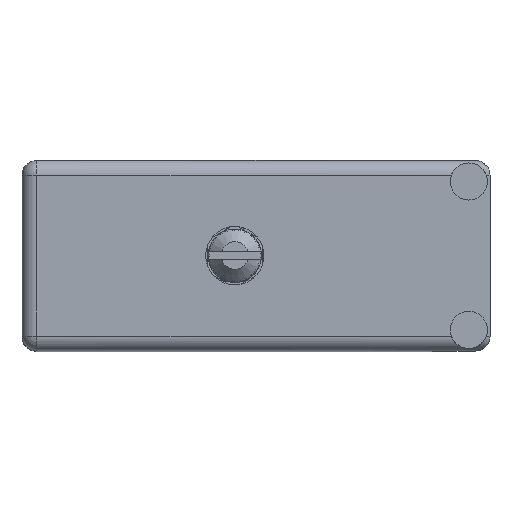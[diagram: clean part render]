
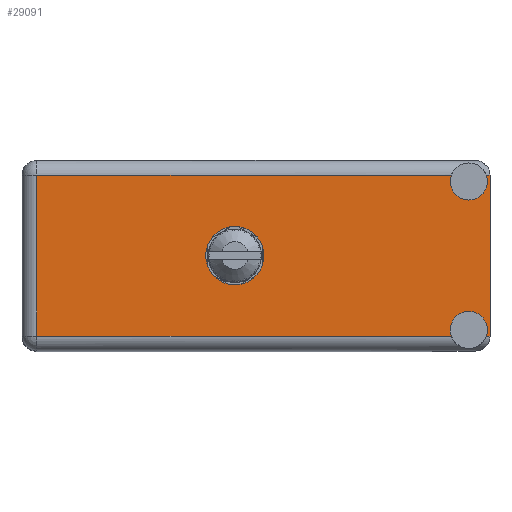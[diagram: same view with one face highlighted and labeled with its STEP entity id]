
A CAD part, top view. The second image highlights one B-rep face of the part: STEP entity #29091.
In plain terms, the highlighted face is planar.
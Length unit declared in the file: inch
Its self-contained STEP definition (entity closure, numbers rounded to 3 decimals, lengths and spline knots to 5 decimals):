
#1974 = DIRECTION ( 'NONE',  ( 0., 1., 0. ) ) ;
#2074 = AXIS2_PLACEMENT_3D ( 'NONE', #16727, #26383, #71237 ) ;
#2833 = VECTOR ( 'NONE', #26097, 39.37008 ) ;
#4726 = VERTEX_POINT ( 'NONE', #74953 ) ;
#4995 = ORIENTED_EDGE ( 'NONE', *, *, #96142, .F. ) ;
#7237 = LINE ( 'NONE', #66171, #75024 ) ;
#10432 = VERTEX_POINT ( 'NONE', #50544 ) ;
#12058 = EDGE_CURVE ( 'NONE', #27234, #93784, #113014, .T. ) ;
#13384 = EDGE_CURVE ( 'NONE', #50701, #30802, #27022, .T. ) ;
#13853 = DIRECTION ( 'NONE',  ( 0., 0., 1. ) ) ;
#14037 = DIRECTION ( 'NONE',  ( 0., 1., 0. ) ) ;
#15318 = AXIS2_PLACEMENT_3D ( 'NONE', #91038, #99223, #46219 ) ;
#15654 = ORIENTED_EDGE ( 'NONE', *, *, #12058, .T. ) ;
#16643 = ORIENTED_EDGE ( 'NONE', *, *, #84531, .F. ) ;
#16688 = DIRECTION ( 'NONE',  ( 0., 1., 0. ) ) ;
#16727 = CARTESIAN_POINT ( 'NONE',  ( 1.104, 1.466, 0.35 ) ) ;
#21860 = CIRCLE ( 'NONE', #15318, 0.1375 ) ;
#23743 = CARTESIAN_POINT ( 'NONE',  ( -1.004, 1.466, -0.4495 ) ) ;
#23768 = ORIENTED_EDGE ( 'NONE', *, *, #49621, .T. ) ;
#25210 = CARTESIAN_POINT ( 'NONE',  ( 1.104, 1.466, -0.35 ) ) ;
#25871 = CARTESIAN_POINT ( 'NONE',  ( -0.934, 1.466, -0.4495 ) ) ;
#25935 = CARTESIAN_POINT ( 'NONE',  ( 1.104, 1.466, -0.2625 ) ) ;
#26097 = DIRECTION ( 'NONE',  ( 1., 0., 0. ) ) ;
#26221 = CARTESIAN_POINT ( 'NONE',  ( -0.934, 1.466, -0.3795 ) ) ;
#26383 = DIRECTION ( 'NONE',  ( 0., 1., 0. ) ) ;
#27022 = LINE ( 'NONE', #32786, #72743 ) ;
#27234 = VERTEX_POINT ( 'NONE', #26221 ) ;
#27567 = CARTESIAN_POINT ( 'NONE',  ( 1.104, 1.466, 0.2625 ) ) ;
#28579 = VECTOR ( 'NONE', #51782, 39.37008 ) ;
#29091 = ADVANCED_FACE ( 'NONE', ( #108712, #38122 ), #93270, .T. ) ;
#30802 = VERTEX_POINT ( 'NONE', #54747 ) ;
#32786 = CARTESIAN_POINT ( 'NONE',  ( 1.204, 1.466, 0.4495 ) ) ;
#32896 = VECTOR ( 'NONE', #70548, 39.37008 ) ;
#34359 = CARTESIAN_POINT ( 'NONE',  ( 1.02162, 1.466, -0.3795 ) ) ;
#35817 = VERTEX_POINT ( 'NONE', #27567 ) ;
#38122 = FACE_OUTER_BOUND ( 'NONE', #89115, .T. ) ;
#42812 = EDGE_CURVE ( 'NONE', #50701, #10432, #85397, .T. ) ;
#43458 = ORIENTED_EDGE ( 'NONE', *, *, #42812, .T. ) ;
#45734 = CARTESIAN_POINT ( 'NONE',  ( 1.104, 1.466, -0.35 ) ) ;
#46219 = DIRECTION ( 'NONE',  ( 0., 0., 1. ) ) ;
#46503 = DIRECTION ( 'NONE',  ( 0., 0., 1. ) ) ;
#47598 = ORIENTED_EDGE ( 'NONE', *, *, #64416, .F. ) ;
#47938 = CARTESIAN_POINT ( 'NONE',  ( -1.004, 1.466, -0.3795 ) ) ;
#48290 = CARTESIAN_POINT ( 'NONE',  ( 0., 1.466, 0. ) ) ;
#49621 = EDGE_CURVE ( 'NONE', #76643, #30802, #7237, .T. ) ;
#49667 = CIRCLE ( 'NONE', #70231, 0.0875 ) ;
#50544 = CARTESIAN_POINT ( 'NONE',  ( 1.18638, 1.466, -0.3795 ) ) ;
#50701 = VERTEX_POINT ( 'NONE', #98220 ) ;
#50771 = EDGE_CURVE ( 'NONE', #72737, #27234, #77562, .T. ) ;
#51782 = DIRECTION ( 'NONE',  ( 0., 0., 1. ) ) ;
#52254 = DIRECTION ( 'NONE',  ( 0., 0., 1. ) ) ;
#53414 = AXIS2_PLACEMENT_3D ( 'NONE', #25210, #16688, #52254 ) ;
#54747 = CARTESIAN_POINT ( 'NONE',  ( 1.204, 1.466, 0.3795 ) ) ;
#58429 = EDGE_LOOP ( 'NONE', ( #47598, #16643 ) ) ;
#58536 = ORIENTED_EDGE ( 'NONE', *, *, #80301, .F. ) ;
#58935 = AXIS2_PLACEMENT_3D ( 'NONE', #23743, #14037, #66215 ) ;
#59672 = CARTESIAN_POINT ( 'NONE',  ( 1.104, 1.466, 0.35 ) ) ;
#60513 = CARTESIAN_POINT ( 'NONE',  ( -0.934, 1.466, 0.3795 ) ) ;
#60664 = EDGE_CURVE ( 'NONE', #72737, #86645, #85470, .T. ) ;
#60845 = CARTESIAN_POINT ( 'NONE',  ( -1.004, 1.466, -0.3795 ) ) ;
#61285 = ORIENTED_EDGE ( 'NONE', *, *, #50771, .T. ) ;
#64218 = ORIENTED_EDGE ( 'NONE', *, *, #60664, .F. ) ;
#64416 = EDGE_CURVE ( 'NONE', #4726, #91240, #21860, .T. ) ;
#65159 = VERTEX_POINT ( 'NONE', #111697 ) ;
#65489 = CIRCLE ( 'NONE', #89573, 0.0875 ) ;
#66171 = CARTESIAN_POINT ( 'NONE',  ( 1.204, 1.466, 0.3795 ) ) ;
#66215 = DIRECTION ( 'NONE',  ( -1., 0., 0. ) ) ;
#67872 = CARTESIAN_POINT ( 'NONE',  ( 1.18638, 1.466, 0.3795 ) ) ;
#70231 = AXIS2_PLACEMENT_3D ( 'NONE', #45734, #1974, #46503 ) ;
#70548 = DIRECTION ( 'NONE',  ( -1., 0., 0. ) ) ;
#71237 = DIRECTION ( 'NONE',  ( 0., 0., 1. ) ) ;
#72737 = VERTEX_POINT ( 'NONE', #34359 ) ;
#72743 = VECTOR ( 'NONE', #111673, 39.37008 ) ;
#73062 = EDGE_CURVE ( 'NONE', #86645, #10432, #49667, .T. ) ;
#73813 = DIRECTION ( 'NONE',  ( -1., 0., 0. ) ) ;
#74953 = CARTESIAN_POINT ( 'NONE',  ( 0., 1.466, 0.1375 ) ) ;
#75024 = VECTOR ( 'NONE', #101817, 39.37008 ) ;
#76643 = VERTEX_POINT ( 'NONE', #67872 ) ;
#77562 = LINE ( 'NONE', #47938, #112245 ) ;
#77826 = CIRCLE ( 'NONE', #2074, 0.0875 ) ;
#80301 = EDGE_CURVE ( 'NONE', #35817, #65159, #77826, .T. ) ;
#84144 = DIRECTION ( 'NONE',  ( 0., 1., 0. ) ) ;
#84531 = EDGE_CURVE ( 'NONE', #91240, #4726, #87142, .T. ) ;
#85397 = LINE ( 'NONE', #60845, #32896 ) ;
#85470 = CIRCLE ( 'NONE', #53414, 0.0875 ) ;
#86298 = AXIS2_PLACEMENT_3D ( 'NONE', #48290, #84144, #13853 ) ;
#86645 = VERTEX_POINT ( 'NONE', #25935 ) ;
#87142 = CIRCLE ( 'NONE', #86298, 0.1375 ) ;
#87782 = ORIENTED_EDGE ( 'NONE', *, *, #108841, .T. ) ;
#88814 = ORIENTED_EDGE ( 'NONE', *, *, #73062, .F. ) ;
#89115 = EDGE_LOOP ( 'NONE', ( #87782, #58536, #4995, #23768, #106826, #43458, #88814, #64218, #61285, #15654 ) ) ;
#89573 = AXIS2_PLACEMENT_3D ( 'NONE', #59672, #104221, #112271 ) ;
#91038 = CARTESIAN_POINT ( 'NONE',  ( 0., 1.466, 0. ) ) ;
#91240 = VERTEX_POINT ( 'NONE', #101767 ) ;
#93270 = PLANE ( 'NONE',  #58935 ) ;
#93784 = VERTEX_POINT ( 'NONE', #60513 ) ;
#96142 = EDGE_CURVE ( 'NONE', #76643, #35817, #65489, .T. ) ;
#96820 = CARTESIAN_POINT ( 'NONE',  ( 1.204, 1.466, 0.3795 ) ) ;
#98220 = CARTESIAN_POINT ( 'NONE',  ( 1.204, 1.466, -0.3795 ) ) ;
#98328 = LINE ( 'NONE', #96820, #2833 ) ;
#99223 = DIRECTION ( 'NONE',  ( 0., 1., 0. ) ) ;
#101767 = CARTESIAN_POINT ( 'NONE',  ( 0., 1.466, -0.1375 ) ) ;
#101817 = DIRECTION ( 'NONE',  ( 1., 0., 0. ) ) ;
#104221 = DIRECTION ( 'NONE',  ( 0., 1., 0. ) ) ;
#106826 = ORIENTED_EDGE ( 'NONE', *, *, #13384, .F. ) ;
#108712 = FACE_BOUND ( 'NONE', #58429, .T. ) ;
#108841 = EDGE_CURVE ( 'NONE', #93784, #65159, #98328, .T. ) ;
#111673 = DIRECTION ( 'NONE',  ( 0., 0., 1. ) ) ;
#111697 = CARTESIAN_POINT ( 'NONE',  ( 1.02162, 1.466, 0.3795 ) ) ;
#112245 = VECTOR ( 'NONE', #73813, 39.37008 ) ;
#112271 = DIRECTION ( 'NONE',  ( 0., 0., 1. ) ) ;
#113014 = LINE ( 'NONE', #25871, #28579 ) ;
